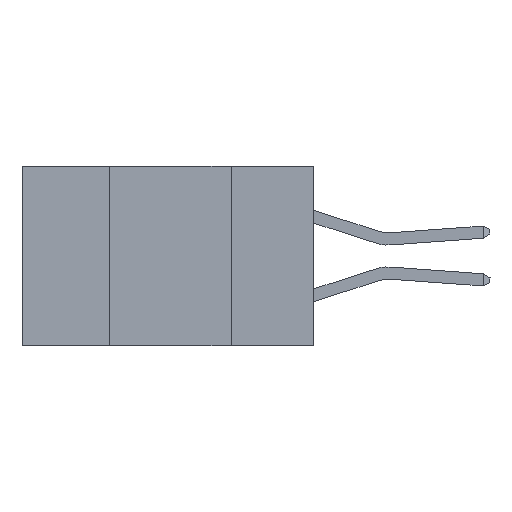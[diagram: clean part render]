
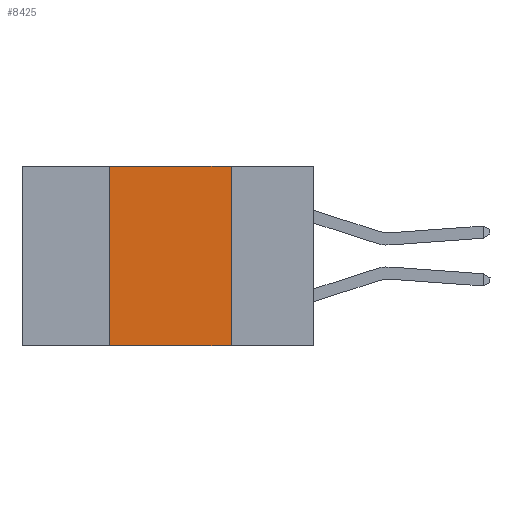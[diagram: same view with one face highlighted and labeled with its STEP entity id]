
A CAD part, left-side view. The second image highlights one B-rep face of the part: STEP entity #8425.
In plain terms, the highlighted planar face has unit normal (-1, 0, 0).
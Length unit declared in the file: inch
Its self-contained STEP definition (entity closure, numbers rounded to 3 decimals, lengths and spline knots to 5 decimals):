
#100 = LINE ( 'NONE', #6380, #3933 ) ;
#406 = EDGE_CURVE ( 'NONE', #20473, #18410, #7021, .T. ) ;
#442 = VECTOR ( 'NONE', #20523, 39.37008 ) ;
#874 = PLANE ( 'NONE',  #19992 ) ;
#937 = DIRECTION ( 'NONE',  ( 0., -1., 0. ) ) ;
#1646 = ORIENTED_EDGE ( 'NONE', *, *, #14651, .F. ) ;
#2397 = CARTESIAN_POINT ( 'NONE',  ( 0., 0.17, 0. ) ) ;
#2724 = CARTESIAN_POINT ( 'NONE',  ( 0., 0.17, -0.37 ) ) ;
#3309 = DIRECTION ( 'NONE',  ( 0., 0., 1. ) ) ;
#3933 = VECTOR ( 'NONE', #19596, 39.37008 ) ;
#4193 = DIRECTION ( 'NONE',  ( 0., 0., -1. ) ) ;
#4659 = ORIENTED_EDGE ( 'NONE', *, *, #10300, .T. ) ;
#5602 = FACE_OUTER_BOUND ( 'NONE', #16535, .T. ) ;
#6380 = CARTESIAN_POINT ( 'NONE',  ( 0., 0.6, -0.37 ) ) ;
#7021 = LINE ( 'NONE', #14040, #10450 ) ;
#7865 = ORIENTED_EDGE ( 'NONE', *, *, #406, .F. ) ;
#8425 = ADVANCED_FACE ( 'NONE', ( #5602 ), #874, .F. ) ;
#8521 = VERTEX_POINT ( 'NONE', #2724 ) ;
#8539 = CARTESIAN_POINT ( 'NONE',  ( 0., 0.42, -0.37 ) ) ;
#10158 = EDGE_CURVE ( 'NONE', #18410, #14063, #20244, .T. ) ;
#10300 = EDGE_CURVE ( 'NONE', #20473, #8521, #100, .T. ) ;
#10450 = VECTOR ( 'NONE', #3309, 39.37008 ) ;
#12100 = CARTESIAN_POINT ( 'NONE',  ( 0., 0.42, 0. ) ) ;
#12586 = CARTESIAN_POINT ( 'NONE',  ( 0., 0.6, 0. ) ) ;
#13759 = LINE ( 'NONE', #18938, #442 ) ;
#14040 = CARTESIAN_POINT ( 'NONE',  ( 0., 0.42, 0. ) ) ;
#14063 = VERTEX_POINT ( 'NONE', #2397 ) ;
#14219 = DIRECTION ( 'NONE',  ( 1., 0., 0. ) ) ;
#14272 = CARTESIAN_POINT ( 'NONE',  ( 0., 0.6, 0. ) ) ;
#14651 = EDGE_CURVE ( 'NONE', #14063, #8521, #13759, .T. ) ;
#15936 = VECTOR ( 'NONE', #937, 39.37008 ) ;
#16535 = EDGE_LOOP ( 'NONE', ( #1646, #18557, #7865, #4659 ) ) ;
#18410 = VERTEX_POINT ( 'NONE', #12100 ) ;
#18557 = ORIENTED_EDGE ( 'NONE', *, *, #10158, .F. ) ;
#18938 = CARTESIAN_POINT ( 'NONE',  ( 0., 0.17, 0. ) ) ;
#19596 = DIRECTION ( 'NONE',  ( 0., -1., 0. ) ) ;
#19992 = AXIS2_PLACEMENT_3D ( 'NONE', #12586, #14219, #4193 ) ;
#20244 = LINE ( 'NONE', #14272, #15936 ) ;
#20473 = VERTEX_POINT ( 'NONE', #8539 ) ;
#20523 = DIRECTION ( 'NONE',  ( 0., 0., -1. ) ) ;
